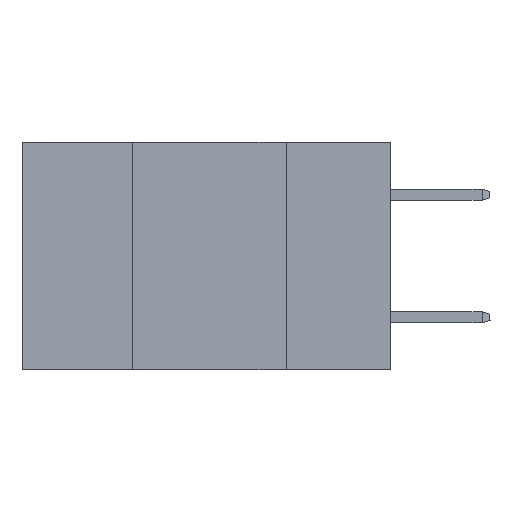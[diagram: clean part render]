
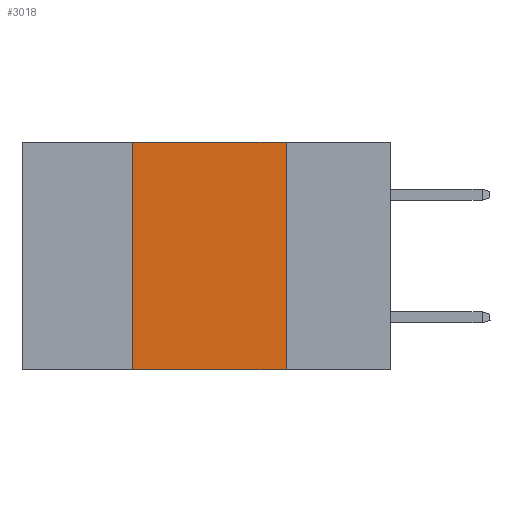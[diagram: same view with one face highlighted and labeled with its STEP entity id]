
A CAD part, left-side view. The second image highlights one B-rep face of the part: STEP entity #3018.
In plain terms, the highlighted planar face has unit normal (-1, 0, 0).
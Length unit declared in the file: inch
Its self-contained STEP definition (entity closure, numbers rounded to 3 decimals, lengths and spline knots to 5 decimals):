
#240 = VERTEX_POINT ( 'NONE', #16741 ) ;
#542 = VECTOR ( 'NONE', #4695, 39.37008 ) ;
#1290 = EDGE_CURVE ( 'NONE', #1871, #240, #14743, .T. ) ;
#1586 = EDGE_CURVE ( 'NONE', #240, #20511, #10277, .T. ) ;
#1871 = VERTEX_POINT ( 'NONE', #12700 ) ;
#2310 = CARTESIAN_POINT ( 'NONE',  ( 0., 0.6, 0. ) ) ;
#3018 = ADVANCED_FACE ( 'NONE', ( #18004 ), #39611, .F. ) ;
#3229 = CARTESIAN_POINT ( 'NONE',  ( 0., 0.6, 0. ) ) ;
#4557 = CARTESIAN_POINT ( 'NONE',  ( 0., 0.17, 0. ) ) ;
#4695 = DIRECTION ( 'NONE',  ( 0., 0., -1. ) ) ;
#4732 = ORIENTED_EDGE ( 'NONE', *, *, #26756, .F. ) ;
#4861 = DIRECTION ( 'NONE',  ( 0., -1., 0. ) ) ;
#6836 = LINE ( 'NONE', #25461, #21474 ) ;
#7665 = ORIENTED_EDGE ( 'NONE', *, *, #19405, .T. ) ;
#9578 = DIRECTION ( 'NONE',  ( 0., 0., 1. ) ) ;
#10277 = LINE ( 'NONE', #4557, #542 ) ;
#12700 = CARTESIAN_POINT ( 'NONE',  ( 0., 0.42, 0. ) ) ;
#14743 = LINE ( 'NONE', #3229, #16152 ) ;
#15325 = DIRECTION ( 'NONE',  ( 0., -1., 0. ) ) ;
#15621 = VECTOR ( 'NONE', #4861, 39.37008 ) ;
#15943 = AXIS2_PLACEMENT_3D ( 'NONE', #2310, #24119, #36612 ) ;
#16152 = VECTOR ( 'NONE', #15325, 39.37008 ) ;
#16741 = CARTESIAN_POINT ( 'NONE',  ( 0., 0.17, 0. ) ) ;
#18004 = FACE_OUTER_BOUND ( 'NONE', #26700, .T. ) ;
#19405 = EDGE_CURVE ( 'NONE', #40280, #20511, #29796, .T. ) ;
#20511 = VERTEX_POINT ( 'NONE', #27863 ) ;
#21474 = VECTOR ( 'NONE', #9578, 39.37008 ) ;
#24119 = DIRECTION ( 'NONE',  ( 1., 0., 0. ) ) ;
#25461 = CARTESIAN_POINT ( 'NONE',  ( 0., 0.42, 0. ) ) ;
#26700 = EDGE_LOOP ( 'NONE', ( #38861, #39971, #4732, #7665 ) ) ;
#26756 = EDGE_CURVE ( 'NONE', #40280, #1871, #6836, .T. ) ;
#27863 = CARTESIAN_POINT ( 'NONE',  ( 0., 0.17, -0.37 ) ) ;
#29796 = LINE ( 'NONE', #38776, #15621 ) ;
#36612 = DIRECTION ( 'NONE',  ( 0., 0., -1. ) ) ;
#38776 = CARTESIAN_POINT ( 'NONE',  ( 0., 0.6, -0.37 ) ) ;
#38861 = ORIENTED_EDGE ( 'NONE', *, *, #1586, .F. ) ;
#38919 = CARTESIAN_POINT ( 'NONE',  ( 0., 0.42, -0.37 ) ) ;
#39611 = PLANE ( 'NONE',  #15943 ) ;
#39971 = ORIENTED_EDGE ( 'NONE', *, *, #1290, .F. ) ;
#40280 = VERTEX_POINT ( 'NONE', #38919 ) ;
